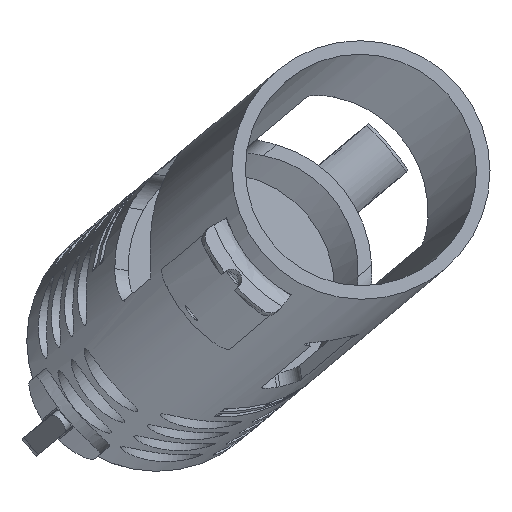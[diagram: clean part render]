
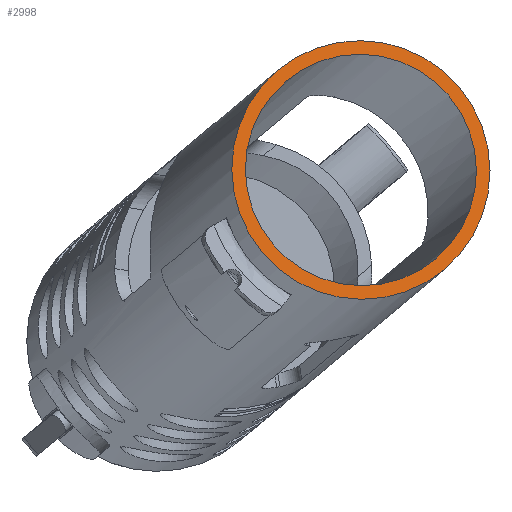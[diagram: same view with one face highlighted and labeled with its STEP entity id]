
A CAD part, front view. The second image highlights one B-rep face of the part: STEP entity #2998.
In plain terms, the highlighted planar face has unit normal (0.107, -0.99, 0.089).
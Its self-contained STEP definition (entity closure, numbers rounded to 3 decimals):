
#71=FACE_BOUND('',#843,.T.);
#510=CIRCLE('',#3197,19.05);
#511=CIRCLE('',#3198,17.05);
#579=PLANE('',#3196);
#683=FACE_OUTER_BOUND('',#842,.T.);
#842=EDGE_LOOP('',(#2264));
#843=EDGE_LOOP('',(#2265));
#1359=VERTEX_POINT('',#6639);
#1360=VERTEX_POINT('',#6641);
#1729=EDGE_CURVE('',#1359,#1359,#510,.T.);
#1730=EDGE_CURVE('',#1360,#1360,#511,.T.);
#2264=ORIENTED_EDGE('',*,*,#1729,.F.);
#2265=ORIENTED_EDGE('',*,*,#1730,.F.);
#2998=ADVANCED_FACE('',(#683,#71),#579,.F.);
#3196=AXIS2_PLACEMENT_3D('',#6638,#3585,#3586);
#3197=AXIS2_PLACEMENT_3D('',#6640,#3587,#3588);
#3198=AXIS2_PLACEMENT_3D('',#6642,#3589,#3590);
#3585=DIRECTION('center_axis',(-0.107,0.99,-0.089));
#3586=DIRECTION('ref_axis',(0.859,0.137,0.494));
#3587=DIRECTION('center_axis',(-0.107,0.99,-0.089));
#3588=DIRECTION('ref_axis',(0.501,-0.024,-0.865));
#3589=DIRECTION('center_axis',(0.107,-0.99,0.089));
#3590=DIRECTION('ref_axis',(-0.501,0.024,0.865));
#6638=CARTESIAN_POINT('Origin',(-163.817,724.662,-138.7));
#6639=CARTESIAN_POINT('',(-173.366,725.123,-122.223));
#6640=CARTESIAN_POINT('Origin',(-163.817,724.662,-138.7));
#6641=CARTESIAN_POINT('',(-155.27,724.25,-153.447));
#6642=CARTESIAN_POINT('Origin',(-163.817,724.662,-138.7));
